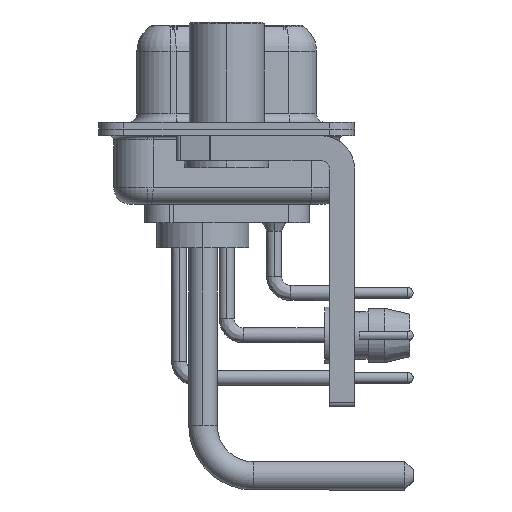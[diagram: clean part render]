
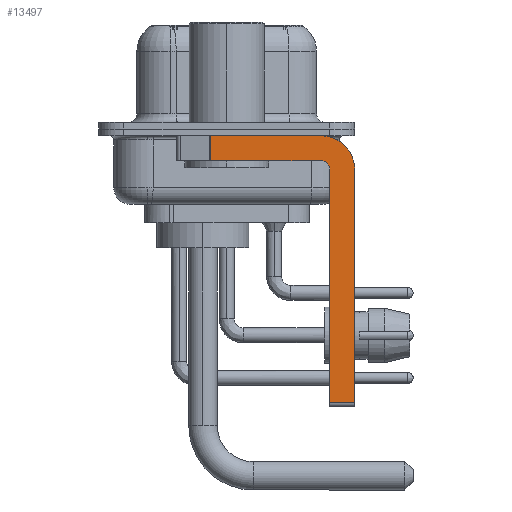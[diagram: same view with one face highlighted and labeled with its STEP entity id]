
A CAD part, left-side view. The second image highlights one B-rep face of the part: STEP entity #13497.
In plain terms, the highlighted planar face has unit normal (-1, 0, 0).
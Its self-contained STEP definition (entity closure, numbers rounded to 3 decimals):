
#334 = FACE_OUTER_BOUND ( 'NONE', #25567, .T. ) ;
#1155 = CARTESIAN_POINT ( 'NONE',  ( -2.9, 3., -0.4 ) ) ;
#2413 = CARTESIAN_POINT ( 'NONE',  ( -2.9, -5.65, -2.4 ) ) ;
#3304 = DIRECTION ( 'NONE',  ( 0., 0., 1. ) ) ;
#3495 = CARTESIAN_POINT ( 'NONE',  ( -2.9, 0.978, -0.4 ) ) ;
#3758 = DIRECTION ( 'NONE',  ( 0., 0., -1. ) ) ;
#4630 = DIRECTION ( 'NONE',  ( 0., -1., 0. ) ) ;
#4775 = VERTEX_POINT ( 'NONE', #22434 ) ;
#4788 = ORIENTED_EDGE ( 'NONE', *, *, #26744, .F. ) ;
#5999 = LINE ( 'NONE', #31530, #14375 ) ;
#6337 = VECTOR ( 'NONE', #29076, 1000. ) ;
#6527 = CARTESIAN_POINT ( 'NONE',  ( -2.9, -5.65, -1.9 ) ) ;
#6545 = CARTESIAN_POINT ( 'NONE',  ( -2.9, -5.65, -2.4 ) ) ;
#6711 = DIRECTION ( 'NONE',  ( 0., 1., 0. ) ) ;
#7446 = VECTOR ( 'NONE', #4630, 1000. ) ;
#7497 = ORIENTED_EDGE ( 'NONE', *, *, #27830, .F. ) ;
#8100 = DIRECTION ( 'NONE',  ( 0., 0., 1. ) ) ;
#8494 = AXIS2_PLACEMENT_3D ( 'NONE', #6545, #26049, #11499 ) ;
#8638 = CARTESIAN_POINT ( 'NONE',  ( -2.9, -6.15, -16.6 ) ) ;
#8930 = DIRECTION ( 'NONE',  ( 0., 0., -1. ) ) ;
#9265 = LINE ( 'NONE', #23272, #35998 ) ;
#9686 = CARTESIAN_POINT ( 'NONE',  ( -2.9, -7.65, -2.4 ) ) ;
#10135 = LINE ( 'NONE', #1155, #6337 ) ;
#11058 = CIRCLE ( 'NONE', #16300, 2. ) ;
#11499 = DIRECTION ( 'NONE',  ( 0., 0., -1. ) ) ;
#11918 = ORIENTED_EDGE ( 'NONE', *, *, #20972, .F. ) ;
#11985 = VERTEX_POINT ( 'NONE', #14511 ) ;
#13028 = ORIENTED_EDGE ( 'NONE', *, *, #17292, .T. ) ;
#13073 = VERTEX_POINT ( 'NONE', #9686 ) ;
#13428 = AXIS2_PLACEMENT_3D ( 'NONE', #32712, #29984, #8100 ) ;
#13497 = ADVANCED_FACE ( 'NONE', ( #334 ), #19841, .F. ) ;
#13577 = DIRECTION ( 'NONE',  ( 1., 0., 0. ) ) ;
#13788 = CARTESIAN_POINT ( 'NONE',  ( -2.9, -7.65, -16.35 ) ) ;
#14375 = VECTOR ( 'NONE', #8930, 1000. ) ;
#14378 = VECTOR ( 'NONE', #6711, 1000. ) ;
#14511 = CARTESIAN_POINT ( 'NONE',  ( -2.9, 0.978, -1.9 ) ) ;
#16300 = AXIS2_PLACEMENT_3D ( 'NONE', #2413, #13577, #27067 ) ;
#16345 = EDGE_CURVE ( 'NONE', #35345, #4775, #10135, .T. ) ;
#16477 = LINE ( 'NONE', #8638, #18347 ) ;
#17037 = VERTEX_POINT ( 'NONE', #24601 ) ;
#17204 = VERTEX_POINT ( 'NONE', #26048 ) ;
#17292 = EDGE_CURVE ( 'NONE', #35345, #11985, #5999, .T. ) ;
#18347 = VECTOR ( 'NONE', #3304, 1000. ) ;
#18672 = LINE ( 'NONE', #29632, #7446 ) ;
#19283 = ORIENTED_EDGE ( 'NONE', *, *, #21110, .F. ) ;
#19841 = PLANE ( 'NONE',  #8494 ) ;
#20972 = EDGE_CURVE ( 'NONE', #4775, #13073, #11058, .T. ) ;
#21110 = EDGE_CURVE ( 'NONE', #34318, #17204, #32628, .T. ) ;
#22434 = CARTESIAN_POINT ( 'NONE',  ( -2.9, -5.65, -0.4 ) ) ;
#23272 = CARTESIAN_POINT ( 'NONE',  ( -2.9, -7.65, -2.4 ) ) ;
#24601 = CARTESIAN_POINT ( 'NONE',  ( -2.9, -6.15, -16.35 ) ) ;
#24642 = ORIENTED_EDGE ( 'NONE', *, *, #29941, .F. ) ;
#25488 = LINE ( 'NONE', #6527, #14378 ) ;
#25567 = EDGE_LOOP ( 'NONE', ( #26085, #13028, #7497, #19283, #4788, #32517, #24642, #11918 ) ) ;
#26048 = CARTESIAN_POINT ( 'NONE',  ( -2.9, -5.65, -1.9 ) ) ;
#26049 = DIRECTION ( 'NONE',  ( 1., 0., 0. ) ) ;
#26085 = ORIENTED_EDGE ( 'NONE', *, *, #16345, .F. ) ;
#26744 = EDGE_CURVE ( 'NONE', #17037, #34318, #16477, .T. ) ;
#27067 = DIRECTION ( 'NONE',  ( 0., 0., -1. ) ) ;
#27830 = EDGE_CURVE ( 'NONE', #17204, #11985, #25488, .T. ) ;
#28022 = EDGE_CURVE ( 'NONE', #17037, #28870, #18672, .T. ) ;
#28870 = VERTEX_POINT ( 'NONE', #13788 ) ;
#29076 = DIRECTION ( 'NONE',  ( 0., -1., 0. ) ) ;
#29632 = CARTESIAN_POINT ( 'NONE',  ( -2.9, -5.65, -16.35 ) ) ;
#29941 = EDGE_CURVE ( 'NONE', #13073, #28870, #9265, .T. ) ;
#29984 = DIRECTION ( 'NONE',  ( -1., 0., 0. ) ) ;
#31530 = CARTESIAN_POINT ( 'NONE',  ( -2.9, 0.978, -1.9 ) ) ;
#32517 = ORIENTED_EDGE ( 'NONE', *, *, #28022, .T. ) ;
#32523 = CARTESIAN_POINT ( 'NONE',  ( -2.9, -6.15, -2.4 ) ) ;
#32628 = CIRCLE ( 'NONE', #13428, 0.5 ) ;
#32712 = CARTESIAN_POINT ( 'NONE',  ( -2.9, -5.65, -2.4 ) ) ;
#34318 = VERTEX_POINT ( 'NONE', #32523 ) ;
#35345 = VERTEX_POINT ( 'NONE', #3495 ) ;
#35998 = VECTOR ( 'NONE', #3758, 1000. ) ;
